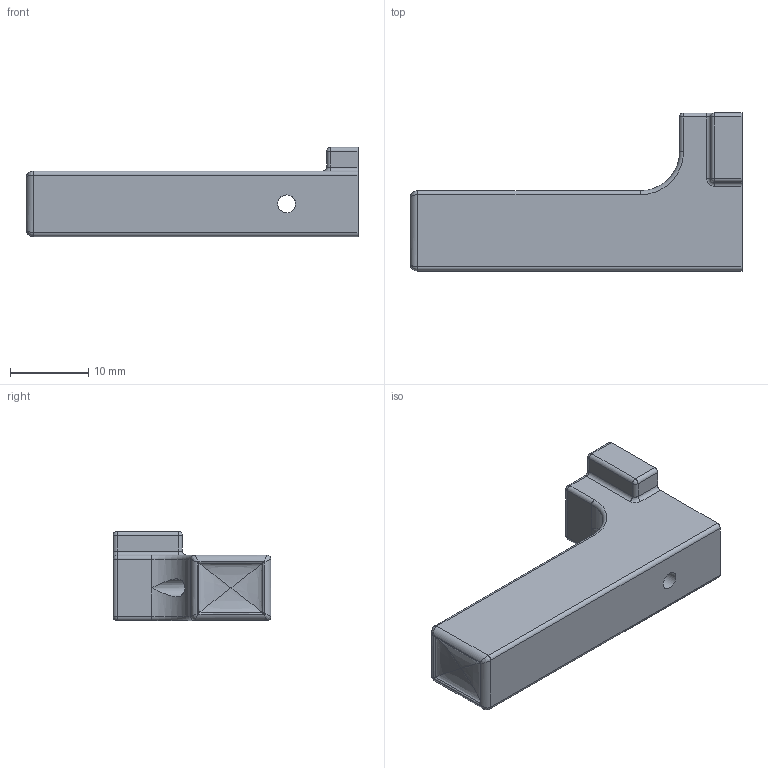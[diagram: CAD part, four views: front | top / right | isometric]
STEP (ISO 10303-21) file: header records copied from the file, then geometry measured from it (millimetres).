
FILE_DESCRIPTION(/* description */ (''),/* implementation_level */ '2;1');
FILE_NAME(/* author */ (''),/* organization */ (''),/* preprocessor_version */ 'ST-DEVELOPER v18.1',/* originating_system */ 'Autodesk Translation Framework v9.3.0.1241',/* authorisation */ '');
FILE_SCHEMA (('AUTOMOTIVE_DESIGN { 1 0 10303 214 3 1 1 }'));
Length unit declared in the file: inch
Products named in the file (1): beretta mag release
Bounding box: 42.36 x 20.15 x 11.38 mm (x, y, z)
Volume: 4303 mm3; surface area: 2211.1 mm2
Topology: 1 solids, 1 shells, 62 faces, 154 edges, 90 vertices
Faces by surface type: cylinder 23, bspline 20, plane 11, sphere 4, torus 4
Full cylindrical faces by diameter (mm): 2.286 x2
Entity records: 2300 total; most frequent: CARTESIAN_POINT 925, ORIENTED_EDGE 300, DIRECTION 247, EDGE_CURVE 150, AXIS2_PLACEMENT_3D 100, VERTEX_POINT 90, EDGE_LOOP 64, FACE_OUTER_BOUND 62
